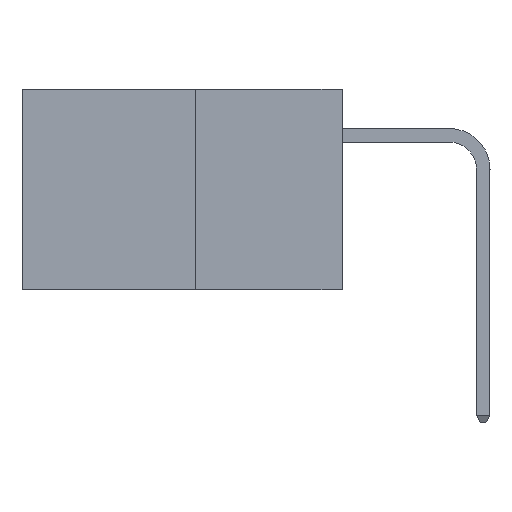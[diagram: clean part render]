
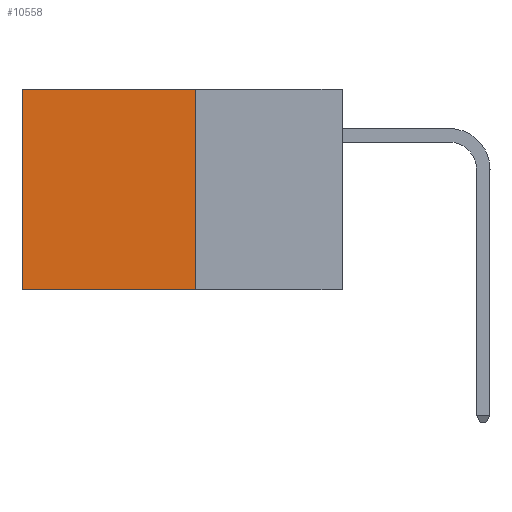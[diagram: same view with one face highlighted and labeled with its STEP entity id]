
A CAD part, left-side view. The second image highlights one B-rep face of the part: STEP entity #10558.
In plain terms, the highlighted planar face has unit normal (-1, 0, 0).
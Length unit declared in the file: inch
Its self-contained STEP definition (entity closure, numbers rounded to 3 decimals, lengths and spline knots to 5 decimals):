
#305 = AXIS2_PLACEMENT_3D ( 'NONE', #11332, #1173, #11393 ) ;
#1173 = DIRECTION ( 'NONE',  ( 1., 0., 0. ) ) ;
#2754 = LINE ( 'NONE', #6155, #6246 ) ;
#2815 = EDGE_LOOP ( 'NONE', ( #7856, #3301, #7772, #6330 ) ) ;
#3301 = ORIENTED_EDGE ( 'NONE', *, *, #17335, .F. ) ;
#3585 = DIRECTION ( 'NONE',  ( 0., 1., 0. ) ) ;
#4658 = DIRECTION ( 'NONE',  ( 0., 0., -1. ) ) ;
#5561 = CARTESIAN_POINT ( 'NONE',  ( 0.277, 0.27, -0.37 ) ) ;
#5684 = FACE_OUTER_BOUND ( 'NONE', #2815, .T. ) ;
#6015 = CARTESIAN_POINT ( 'NONE',  ( 0.277, 0.27, 0. ) ) ;
#6155 = CARTESIAN_POINT ( 'NONE',  ( 0.277, 0.59, -0.37 ) ) ;
#6228 = CARTESIAN_POINT ( 'NONE',  ( 0.277, 0.27, -0.37 ) ) ;
#6246 = VECTOR ( 'NONE', #14754, 39.37008 ) ;
#6330 = ORIENTED_EDGE ( 'NONE', *, *, #15320, .T. ) ;
#6698 = VECTOR ( 'NONE', #3585, 39.37008 ) ;
#6970 = VERTEX_POINT ( 'NONE', #18642 ) ;
#7772 = ORIENTED_EDGE ( 'NONE', *, *, #10129, .F. ) ;
#7856 = ORIENTED_EDGE ( 'NONE', *, *, #14349, .T. ) ;
#8406 = VERTEX_POINT ( 'NONE', #13439 ) ;
#8635 = VECTOR ( 'NONE', #4658, 39.37008 ) ;
#9638 = CARTESIAN_POINT ( 'NONE',  ( 0.277, 0.59, -0.37 ) ) ;
#9913 = PLANE ( 'NONE',  #305 ) ;
#10129 = EDGE_CURVE ( 'NONE', #6970, #18631, #16213, .T. ) ;
#10558 = ADVANCED_FACE ( 'NONE', ( #5684 ), #9913, .F. ) ;
#11332 = CARTESIAN_POINT ( 'NONE',  ( 0.277, 0.27, -0.37 ) ) ;
#11393 = DIRECTION ( 'NONE',  ( 0., 0., -1. ) ) ;
#11833 = DIRECTION ( 'NONE',  ( 0., 1., 0. ) ) ;
#12346 = CARTESIAN_POINT ( 'NONE',  ( 0.277, 0.27, -0.37 ) ) ;
#13439 = CARTESIAN_POINT ( 'NONE',  ( 0.277, 0.59, 0. ) ) ;
#14349 = EDGE_CURVE ( 'NONE', #8406, #17949, #2754, .T. ) ;
#14754 = DIRECTION ( 'NONE',  ( 0., 0., -1. ) ) ;
#15320 = EDGE_CURVE ( 'NONE', #6970, #8406, #15940, .T. ) ;
#15506 = VECTOR ( 'NONE', #11833, 39.37008 ) ;
#15940 = LINE ( 'NONE', #6015, #15506 ) ;
#16213 = LINE ( 'NONE', #6228, #8635 ) ;
#17335 = EDGE_CURVE ( 'NONE', #18631, #17949, #17593, .T. ) ;
#17593 = LINE ( 'NONE', #12346, #6698 ) ;
#17949 = VERTEX_POINT ( 'NONE', #9638 ) ;
#18631 = VERTEX_POINT ( 'NONE', #5561 ) ;
#18642 = CARTESIAN_POINT ( 'NONE',  ( 0.277, 0.27, 0. ) ) ;
